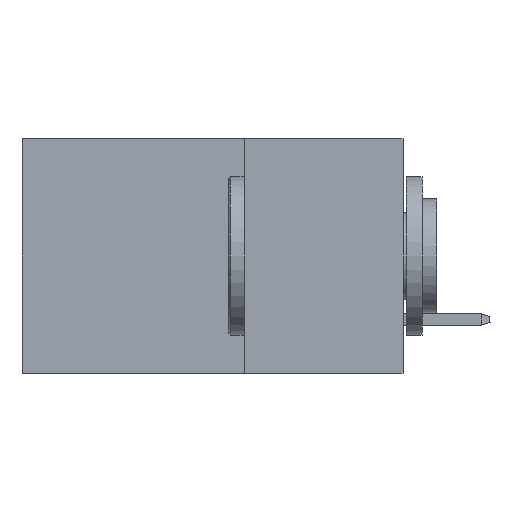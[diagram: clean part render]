
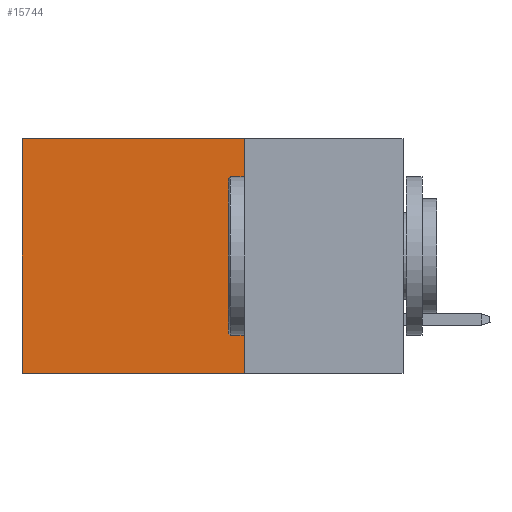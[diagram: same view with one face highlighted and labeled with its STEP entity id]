
A CAD part, left-side view. The second image highlights one B-rep face of the part: STEP entity #15744.
In plain terms, the highlighted planar face has unit normal (-1, 0, 0).
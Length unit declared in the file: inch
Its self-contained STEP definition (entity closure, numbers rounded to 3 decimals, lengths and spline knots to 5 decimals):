
#279 = CARTESIAN_POINT ( 'NONE',  ( 0.2875, 0.25, -0.37 ) ) ;
#472 = LINE ( 'NONE', #14624, #12546 ) ;
#605 = ORIENTED_EDGE ( 'NONE', *, *, #822, .T. ) ;
#822 = EDGE_CURVE ( 'NONE', #9145, #8790, #472, .T. ) ;
#1735 = ORIENTED_EDGE ( 'NONE', *, *, #19200, .F. ) ;
#2690 = CARTESIAN_POINT ( 'NONE',  ( 0.2875, 0.25, -0.37 ) ) ;
#3635 = EDGE_CURVE ( 'NONE', #12644, #8150, #10052, .T. ) ;
#3723 = DIRECTION ( 'NONE',  ( 0., 0., -1. ) ) ;
#4890 = DIRECTION ( 'NONE',  ( 0., 0., -1. ) ) ;
#5590 = LINE ( 'NONE', #9054, #6024 ) ;
#6024 = VECTOR ( 'NONE', #19797, 39.37008 ) ;
#7079 = VECTOR ( 'NONE', #3723, 39.37008 ) ;
#8150 = VERTEX_POINT ( 'NONE', #2690 ) ;
#8617 = VECTOR ( 'NONE', #10984, 39.37008 ) ;
#8790 = VERTEX_POINT ( 'NONE', #19211 ) ;
#9054 = CARTESIAN_POINT ( 'NONE',  ( 0.2875, 0.25, 0. ) ) ;
#9145 = VERTEX_POINT ( 'NONE', #9956 ) ;
#9941 = ORIENTED_EDGE ( 'NONE', *, *, #3635, .F. ) ;
#9956 = CARTESIAN_POINT ( 'NONE',  ( 0.2875, 0.6, 0. ) ) ;
#10052 = LINE ( 'NONE', #13213, #7079 ) ;
#10984 = DIRECTION ( 'NONE',  ( 0., 1., 0. ) ) ;
#12546 = VECTOR ( 'NONE', #12998, 39.37008 ) ;
#12632 = DIRECTION ( 'NONE',  ( 1., 0., 0. ) ) ;
#12644 = VERTEX_POINT ( 'NONE', #18254 ) ;
#12998 = DIRECTION ( 'NONE',  ( 0., 0., -1. ) ) ;
#13213 = CARTESIAN_POINT ( 'NONE',  ( 0.2875, 0.25, 0. ) ) ;
#14033 = LINE ( 'NONE', #279, #8617 ) ;
#14062 = FACE_OUTER_BOUND ( 'NONE', #15814, .T. ) ;
#14168 = ORIENTED_EDGE ( 'NONE', *, *, #19133, .T. ) ;
#14355 = CARTESIAN_POINT ( 'NONE',  ( 0.2875, 0.25, 0. ) ) ;
#14624 = CARTESIAN_POINT ( 'NONE',  ( 0.2875, 0.6, 0. ) ) ;
#15686 = AXIS2_PLACEMENT_3D ( 'NONE', #14355, #12632, #4890 ) ;
#15744 = ADVANCED_FACE ( 'NONE', ( #14062 ), #17175, .F. ) ;
#15814 = EDGE_LOOP ( 'NONE', ( #605, #1735, #9941, #14168 ) ) ;
#17175 = PLANE ( 'NONE',  #15686 ) ;
#18254 = CARTESIAN_POINT ( 'NONE',  ( 0.2875, 0.25, 0. ) ) ;
#19133 = EDGE_CURVE ( 'NONE', #12644, #9145, #5590, .T. ) ;
#19200 = EDGE_CURVE ( 'NONE', #8150, #8790, #14033, .T. ) ;
#19211 = CARTESIAN_POINT ( 'NONE',  ( 0.2875, 0.6, -0.37 ) ) ;
#19797 = DIRECTION ( 'NONE',  ( 0., 1., 0. ) ) ;
